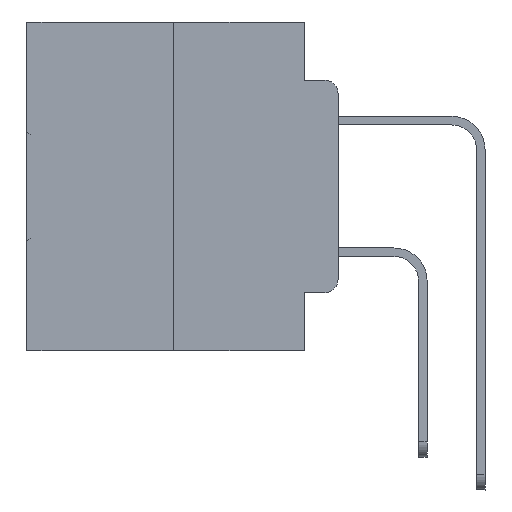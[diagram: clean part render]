
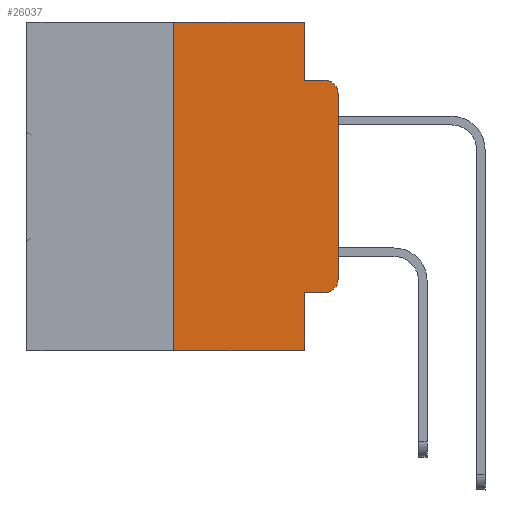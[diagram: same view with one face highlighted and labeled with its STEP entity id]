
A CAD part, left-side view. The second image highlights one B-rep face of the part: STEP entity #26037.
In plain terms, the highlighted planar face has unit normal (-1, 0, 0).
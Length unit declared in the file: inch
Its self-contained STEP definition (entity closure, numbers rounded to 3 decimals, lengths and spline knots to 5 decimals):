
#638 = LINE ( 'NONE', #13559, #16354 ) ;
#743 = AXIS2_PLACEMENT_3D ( 'NONE', #21217, #13219, #16207 ) ;
#810 = DIRECTION ( 'NONE',  ( 0., -1., 0. ) ) ;
#1267 = VECTOR ( 'NONE', #15344, 39.37008 ) ;
#1302 = PLANE ( 'NONE',  #9823 ) ;
#1558 = VERTEX_POINT ( 'NONE', #15154 ) ;
#1798 = EDGE_LOOP ( 'NONE', ( #23145, #11739, #18807, #9022, #23416, #11390, #23982, #5834, #31697, #2458 ) ) ;
#1821 = CIRCLE ( 'NONE', #743, 0.02 ) ;
#1914 = LINE ( 'NONE', #29894, #13023 ) ;
#2458 = ORIENTED_EDGE ( 'NONE', *, *, #25246, .T. ) ;
#2787 = CARTESIAN_POINT ( 'NONE',  ( 0., 0.25, 0. ) ) ;
#2952 = VERTEX_POINT ( 'NONE', #4492 ) ;
#2981 = FACE_OUTER_BOUND ( 'NONE', #1798, .T. ) ;
#3135 = DIRECTION ( 'NONE',  ( 0., 0., 1. ) ) ;
#3433 = DIRECTION ( 'NONE',  ( 0., 0., -1. ) ) ;
#4492 = CARTESIAN_POINT ( 'NONE',  ( 0., 0.25, -0.5 ) ) ;
#4893 = LINE ( 'NONE', #20300, #27802 ) ;
#5132 = LINE ( 'NONE', #7322, #1267 ) ;
#5655 = EDGE_CURVE ( 'NONE', #24952, #12932, #28262, .T. ) ;
#5834 = ORIENTED_EDGE ( 'NONE', *, *, #8905, .F. ) ;
#5903 = EDGE_CURVE ( 'NONE', #12932, #10412, #1821, .T. ) ;
#6978 = EDGE_CURVE ( 'NONE', #8330, #23524, #638, .T. ) ;
#7322 = CARTESIAN_POINT ( 'NONE',  ( 0., 0.051, -0.0885 ) ) ;
#8330 = VERTEX_POINT ( 'NONE', #28991 ) ;
#8872 = DIRECTION ( 'NONE',  ( 0., 0., -1. ) ) ;
#8905 = EDGE_CURVE ( 'NONE', #12580, #22743, #4893, .T. ) ;
#9022 = ORIENTED_EDGE ( 'NONE', *, *, #23955, .F. ) ;
#9363 = DIRECTION ( 'NONE',  ( 0., -1., 0. ) ) ;
#9823 = AXIS2_PLACEMENT_3D ( 'NONE', #29284, #11566, #8872 ) ;
#9856 = VECTOR ( 'NONE', #9363, 39.37008 ) ;
#10190 = DIRECTION ( 'NONE',  ( 0., 0., -1. ) ) ;
#10412 = VERTEX_POINT ( 'NONE', #11492 ) ;
#11390 = ORIENTED_EDGE ( 'NONE', *, *, #13336, .F. ) ;
#11492 = CARTESIAN_POINT ( 'NONE',  ( 0., 0.02, -0.0885 ) ) ;
#11563 = CARTESIAN_POINT ( 'NONE',  ( 0., 0.473, -0.5 ) ) ;
#11566 = DIRECTION ( 'NONE',  ( 1., 0., 0. ) ) ;
#11624 = VECTOR ( 'NONE', #3135, 39.37008 ) ;
#11739 = ORIENTED_EDGE ( 'NONE', *, *, #5903, .T. ) ;
#12580 = VERTEX_POINT ( 'NONE', #27000 ) ;
#12932 = VERTEX_POINT ( 'NONE', #20925 ) ;
#13023 = VECTOR ( 'NONE', #25177, 39.37008 ) ;
#13219 = DIRECTION ( 'NONE',  ( -1., 0., 0. ) ) ;
#13336 = EDGE_CURVE ( 'NONE', #2952, #8330, #17899, .T. ) ;
#13512 = LINE ( 'NONE', #26369, #29582 ) ;
#13559 = CARTESIAN_POINT ( 'NONE',  ( 0., 0.473, 0. ) ) ;
#15154 = CARTESIAN_POINT ( 'NONE',  ( 0., 0.02, -0.4115 ) ) ;
#15182 = CARTESIAN_POINT ( 'NONE',  ( 0., 0.02, -0.3915 ) ) ;
#15224 = CARTESIAN_POINT ( 'NONE',  ( 0., 0., 0. ) ) ;
#15344 = DIRECTION ( 'NONE',  ( 0., -1., 0. ) ) ;
#16207 = DIRECTION ( 'NONE',  ( 0., 0., -1. ) ) ;
#16354 = VECTOR ( 'NONE', #810, 39.37008 ) ;
#16551 = LINE ( 'NONE', #11563, #9856 ) ;
#17018 = VERTEX_POINT ( 'NONE', #18669 ) ;
#17899 = LINE ( 'NONE', #2787, #11624 ) ;
#18400 = VECTOR ( 'NONE', #30945, 39.37008 ) ;
#18669 = CARTESIAN_POINT ( 'NONE',  ( 0., 0.051, -0.0885 ) ) ;
#18807 = ORIENTED_EDGE ( 'NONE', *, *, #25167, .F. ) ;
#20300 = CARTESIAN_POINT ( 'NONE',  ( 0., 0.051, 0. ) ) ;
#20925 = CARTESIAN_POINT ( 'NONE',  ( 0., 0., -0.1085 ) ) ;
#21217 = CARTESIAN_POINT ( 'NONE',  ( 0., 0.02, -0.1085 ) ) ;
#22743 = VERTEX_POINT ( 'NONE', #28213 ) ;
#23145 = ORIENTED_EDGE ( 'NONE', *, *, #5655, .T. ) ;
#23416 = ORIENTED_EDGE ( 'NONE', *, *, #6978, .F. ) ;
#23524 = VERTEX_POINT ( 'NONE', #28427 ) ;
#23955 = EDGE_CURVE ( 'NONE', #23524, #17018, #13512, .T. ) ;
#23982 = ORIENTED_EDGE ( 'NONE', *, *, #25135, .T. ) ;
#24185 = EDGE_CURVE ( 'NONE', #12580, #1558, #1914, .T. ) ;
#24952 = VERTEX_POINT ( 'NONE', #28436 ) ;
#25135 = EDGE_CURVE ( 'NONE', #2952, #22743, #16551, .T. ) ;
#25167 = EDGE_CURVE ( 'NONE', #17018, #10412, #5132, .T. ) ;
#25177 = DIRECTION ( 'NONE',  ( 0., -1., 0. ) ) ;
#25246 = EDGE_CURVE ( 'NONE', #1558, #24952, #25276, .T. ) ;
#25276 = CIRCLE ( 'NONE', #27412, 0.02 ) ;
#26037 = ADVANCED_FACE ( 'NONE', ( #2981 ), #1302, .F. ) ;
#26369 = CARTESIAN_POINT ( 'NONE',  ( 0., 0.051, 0. ) ) ;
#27000 = CARTESIAN_POINT ( 'NONE',  ( 0., 0.051, -0.4115 ) ) ;
#27412 = AXIS2_PLACEMENT_3D ( 'NONE', #15182, #27572, #10190 ) ;
#27572 = DIRECTION ( 'NONE',  ( -1., 0., 0. ) ) ;
#27802 = VECTOR ( 'NONE', #32251, 39.37008 ) ;
#28213 = CARTESIAN_POINT ( 'NONE',  ( 0., 0.051, -0.5 ) ) ;
#28262 = LINE ( 'NONE', #15224, #18400 ) ;
#28427 = CARTESIAN_POINT ( 'NONE',  ( 0., 0.051, 0. ) ) ;
#28436 = CARTESIAN_POINT ( 'NONE',  ( 0., 0., -0.3915 ) ) ;
#28991 = CARTESIAN_POINT ( 'NONE',  ( 0., 0.25, 0. ) ) ;
#29284 = CARTESIAN_POINT ( 'NONE',  ( 0., 0.473, 0. ) ) ;
#29582 = VECTOR ( 'NONE', #3433, 39.37008 ) ;
#29894 = CARTESIAN_POINT ( 'NONE',  ( 0., 0.051, -0.4115 ) ) ;
#30945 = DIRECTION ( 'NONE',  ( 0., 0., 1. ) ) ;
#31697 = ORIENTED_EDGE ( 'NONE', *, *, #24185, .T. ) ;
#32251 = DIRECTION ( 'NONE',  ( 0., 0., -1. ) ) ;
